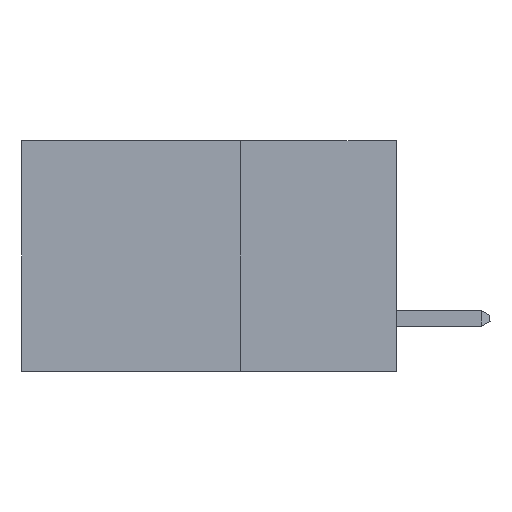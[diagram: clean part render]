
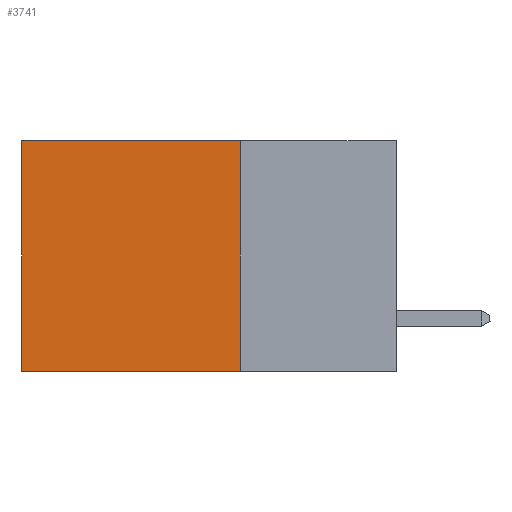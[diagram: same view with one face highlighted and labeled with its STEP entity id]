
A CAD part, left-side view. The second image highlights one B-rep face of the part: STEP entity #3741.
In plain terms, the highlighted planar face has unit normal (-1, 0, 0).
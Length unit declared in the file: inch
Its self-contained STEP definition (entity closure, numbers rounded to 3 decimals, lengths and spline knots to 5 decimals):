
#388 = CARTESIAN_POINT ( 'NONE',  ( 0.298, 0.25, 0. ) ) ;
#2040 = ORIENTED_EDGE ( 'NONE', *, *, #17702, .T. ) ;
#2304 = EDGE_LOOP ( 'NONE', ( #2040, #3414, #9967, #15494 ) ) ;
#2390 = LINE ( 'NONE', #15521, #9855 ) ;
#2538 = EDGE_CURVE ( 'NONE', #14203, #9712, #9596, .T. ) ;
#2580 = VECTOR ( 'NONE', #8804, 39.37008 ) ;
#2617 = VERTEX_POINT ( 'NONE', #10540 ) ;
#3399 = CARTESIAN_POINT ( 'NONE',  ( 0.298, 0.25, 0. ) ) ;
#3414 = ORIENTED_EDGE ( 'NONE', *, *, #7071, .F. ) ;
#3741 = ADVANCED_FACE ( 'NONE', ( #15219 ), #7979, .F. ) ;
#4259 = CARTESIAN_POINT ( 'NONE',  ( 0.298, 0.25, -0.37 ) ) ;
#4371 = CARTESIAN_POINT ( 'NONE',  ( 0.298, 0.25, 0. ) ) ;
#4762 = VERTEX_POINT ( 'NONE', #17290 ) ;
#5967 = AXIS2_PLACEMENT_3D ( 'NONE', #13691, #16552, #8049 ) ;
#7071 = EDGE_CURVE ( 'NONE', #9712, #4762, #12331, .T. ) ;
#7979 = PLANE ( 'NONE',  #5967 ) ;
#8049 = DIRECTION ( 'NONE',  ( 0., 0., -1. ) ) ;
#8804 = DIRECTION ( 'NONE',  ( 0., 1., 0. ) ) ;
#9368 = VECTOR ( 'NONE', #16196, 39.37008 ) ;
#9596 = LINE ( 'NONE', #4371, #9368 ) ;
#9712 = VERTEX_POINT ( 'NONE', #12050 ) ;
#9813 = LINE ( 'NONE', #388, #2580 ) ;
#9855 = VECTOR ( 'NONE', #13984, 39.37008 ) ;
#9967 = ORIENTED_EDGE ( 'NONE', *, *, #2538, .F. ) ;
#10540 = CARTESIAN_POINT ( 'NONE',  ( 0.298, 0.6, 0. ) ) ;
#12050 = CARTESIAN_POINT ( 'NONE',  ( 0.298, 0.25, -0.37 ) ) ;
#12331 = LINE ( 'NONE', #4259, #13647 ) ;
#13647 = VECTOR ( 'NONE', #15687, 39.37008 ) ;
#13691 = CARTESIAN_POINT ( 'NONE',  ( 0.298, 0.25, 0. ) ) ;
#13974 = EDGE_CURVE ( 'NONE', #14203, #2617, #9813, .T. ) ;
#13984 = DIRECTION ( 'NONE',  ( 0., 0., -1. ) ) ;
#14203 = VERTEX_POINT ( 'NONE', #3399 ) ;
#15219 = FACE_OUTER_BOUND ( 'NONE', #2304, .T. ) ;
#15494 = ORIENTED_EDGE ( 'NONE', *, *, #13974, .T. ) ;
#15521 = CARTESIAN_POINT ( 'NONE',  ( 0.298, 0.6, 0. ) ) ;
#15687 = DIRECTION ( 'NONE',  ( 0., 1., 0. ) ) ;
#16196 = DIRECTION ( 'NONE',  ( 0., 0., -1. ) ) ;
#16552 = DIRECTION ( 'NONE',  ( 1., 0., 0. ) ) ;
#17290 = CARTESIAN_POINT ( 'NONE',  ( 0.298, 0.6, -0.37 ) ) ;
#17702 = EDGE_CURVE ( 'NONE', #2617, #4762, #2390, .T. ) ;
